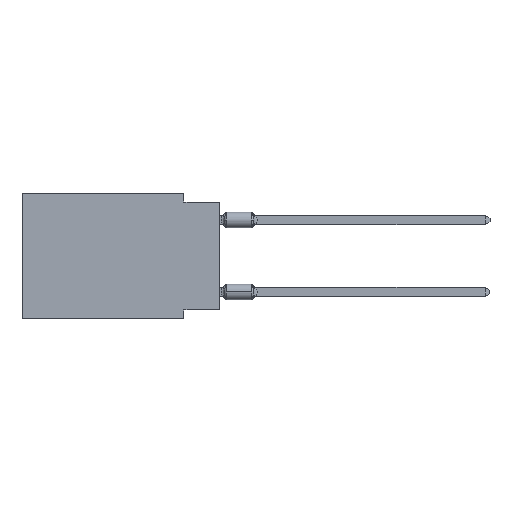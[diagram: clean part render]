
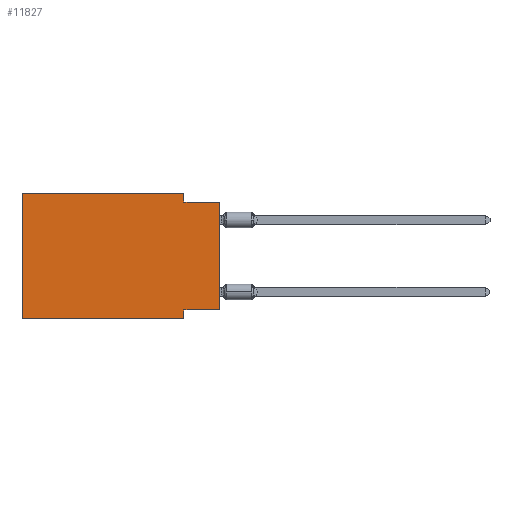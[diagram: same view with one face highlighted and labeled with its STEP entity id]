
A CAD part, left-side view. The second image highlights one B-rep face of the part: STEP entity #11827.
In plain terms, the highlighted planar face has unit normal (-1, 0, 0).
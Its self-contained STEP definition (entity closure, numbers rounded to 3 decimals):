
#53 = CARTESIAN_POINT ( 'NONE',  ( 0., 13.97, -8.89 ) ) ;
#146 = VERTEX_POINT ( 'NONE', #53 ) ;
#529 = VECTOR ( 'NONE', #12722, 1000. ) ;
#570 = EDGE_CURVE ( 'NONE', #146, #2164, #8297, .T. ) ;
#665 = VERTEX_POINT ( 'NONE', #11062 ) ;
#1271 = VERTEX_POINT ( 'NONE', #3717 ) ;
#1348 = DIRECTION ( 'NONE',  ( 1., 0., 0. ) ) ;
#1415 = DIRECTION ( 'NONE',  ( 0., -1., 0. ) ) ;
#1672 = CARTESIAN_POINT ( 'NONE',  ( 0., 13.97, 0. ) ) ;
#2164 = VERTEX_POINT ( 'NONE', #12733 ) ;
#2311 = VECTOR ( 'NONE', #9719, 1000. ) ;
#2412 = LINE ( 'NONE', #4591, #2311 ) ;
#2645 = LINE ( 'NONE', #6367, #4184 ) ;
#2674 = LINE ( 'NONE', #12903, #9382 ) ;
#3642 = EDGE_CURVE ( 'NONE', #1271, #5158, #8462, .T. ) ;
#3644 = ORIENTED_EDGE ( 'NONE', *, *, #3642, .F. ) ;
#3717 = CARTESIAN_POINT ( 'NONE',  ( 0., 2.54, -0.635 ) ) ;
#3760 = VERTEX_POINT ( 'NONE', #14123 ) ;
#4184 = VECTOR ( 'NONE', #7621, 1000. ) ;
#4527 = CARTESIAN_POINT ( 'NONE',  ( 0., 0., -0.635 ) ) ;
#4591 = CARTESIAN_POINT ( 'NONE',  ( 0., 0., -8.255 ) ) ;
#4700 = VECTOR ( 'NONE', #5599, 1000. ) ;
#4794 = PLANE ( 'NONE',  #7384 ) ;
#5110 = VERTEX_POINT ( 'NONE', #15747 ) ;
#5158 = VERTEX_POINT ( 'NONE', #4527 ) ;
#5599 = DIRECTION ( 'NONE',  ( 0., 0., 1. ) ) ;
#5777 = EDGE_CURVE ( 'NONE', #3760, #5110, #2412, .T. ) ;
#5809 = EDGE_CURVE ( 'NONE', #2164, #665, #2645, .T. ) ;
#6367 = CARTESIAN_POINT ( 'NONE',  ( 0., 13.97, 0. ) ) ;
#6410 = VECTOR ( 'NONE', #8345, 1000. ) ;
#6477 = DIRECTION ( 'NONE',  ( 0., 0., -1. ) ) ;
#6592 = ORIENTED_EDGE ( 'NONE', *, *, #5809, .F. ) ;
#7177 = DIRECTION ( 'NONE',  ( 0., 0., -1. ) ) ;
#7247 = EDGE_CURVE ( 'NONE', #5110, #7940, #8609, .T. ) ;
#7384 = AXIS2_PLACEMENT_3D ( 'NONE', #1672, #1348, #6477 ) ;
#7621 = DIRECTION ( 'NONE',  ( 0., -1., 0. ) ) ;
#7730 = ORIENTED_EDGE ( 'NONE', *, *, #16274, .T. ) ;
#7870 = CARTESIAN_POINT ( 'NONE',  ( 0., 0., -0.635 ) ) ;
#7940 = VERTEX_POINT ( 'NONE', #14466 ) ;
#8297 = LINE ( 'NONE', #15973, #4700 ) ;
#8345 = DIRECTION ( 'NONE',  ( 0., 0., 1. ) ) ;
#8462 = LINE ( 'NONE', #7870, #529 ) ;
#8609 = LINE ( 'NONE', #9874, #15190 ) ;
#9001 = ORIENTED_EDGE ( 'NONE', *, *, #7247, .F. ) ;
#9382 = VECTOR ( 'NONE', #1415, 1000. ) ;
#9554 = EDGE_CURVE ( 'NONE', #146, #7940, #2674, .T. ) ;
#9719 = DIRECTION ( 'NONE',  ( 0., 1., 0. ) ) ;
#9874 = CARTESIAN_POINT ( 'NONE',  ( 0., 2.54, -8.89 ) ) ;
#9896 = ORIENTED_EDGE ( 'NONE', *, *, #9554, .T. ) ;
#10508 = LINE ( 'NONE', #11752, #16439 ) ;
#10809 = ORIENTED_EDGE ( 'NONE', *, *, #14642, .F. ) ;
#10993 = EDGE_LOOP ( 'NONE', ( #7730, #3644, #10809, #6592, #15727, #9896, #9001, #13274 ) ) ;
#11062 = CARTESIAN_POINT ( 'NONE',  ( 0., 2.54, 0. ) ) ;
#11752 = CARTESIAN_POINT ( 'NONE',  ( 0., 2.54, 0. ) ) ;
#11827 = ADVANCED_FACE ( 'NONE', ( #16263 ), #4794, .F. ) ;
#12192 = CARTESIAN_POINT ( 'NONE',  ( 0., 0., 0. ) ) ;
#12722 = DIRECTION ( 'NONE',  ( 0., -1., 0. ) ) ;
#12733 = CARTESIAN_POINT ( 'NONE',  ( 0., 13.97, 0. ) ) ;
#12903 = CARTESIAN_POINT ( 'NONE',  ( 0., 13.97, -8.89 ) ) ;
#13152 = DIRECTION ( 'NONE',  ( 0., 0., -1. ) ) ;
#13274 = ORIENTED_EDGE ( 'NONE', *, *, #5777, .F. ) ;
#14123 = CARTESIAN_POINT ( 'NONE',  ( 0., 0., -8.255 ) ) ;
#14347 = LINE ( 'NONE', #12192, #6410 ) ;
#14466 = CARTESIAN_POINT ( 'NONE',  ( 0., 2.54, -8.89 ) ) ;
#14642 = EDGE_CURVE ( 'NONE', #665, #1271, #10508, .T. ) ;
#15190 = VECTOR ( 'NONE', #7177, 1000. ) ;
#15727 = ORIENTED_EDGE ( 'NONE', *, *, #570, .F. ) ;
#15747 = CARTESIAN_POINT ( 'NONE',  ( 0., 2.54, -8.255 ) ) ;
#15973 = CARTESIAN_POINT ( 'NONE',  ( 0., 13.97, 0. ) ) ;
#16263 = FACE_OUTER_BOUND ( 'NONE', #10993, .T. ) ;
#16274 = EDGE_CURVE ( 'NONE', #3760, #5158, #14347, .T. ) ;
#16439 = VECTOR ( 'NONE', #13152, 1000. ) ;
